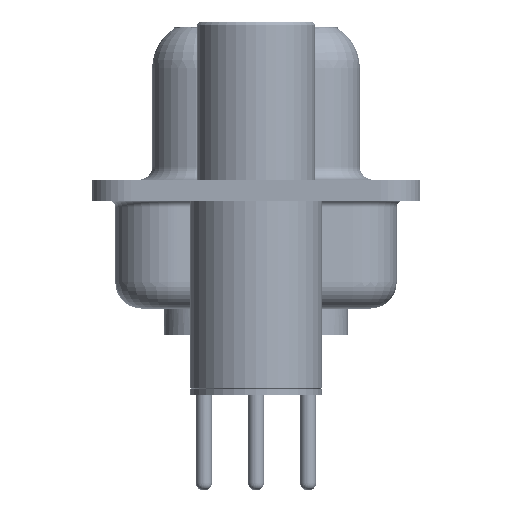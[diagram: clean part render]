
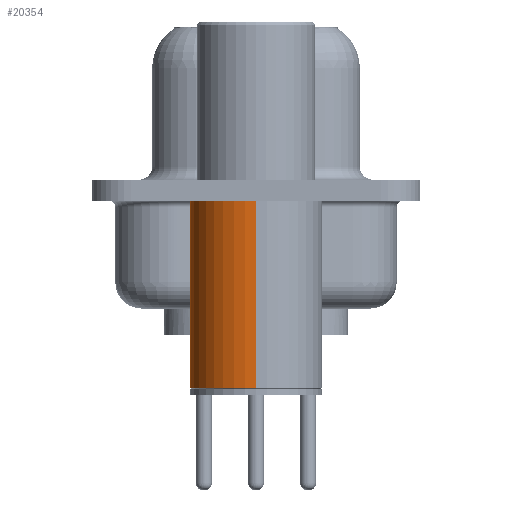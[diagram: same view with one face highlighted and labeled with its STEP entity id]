
A CAD part, left-side view. The second image highlights one B-rep face of the part: STEP entity #20354.
In plain terms, the highlighted cylindrical face has radius 2.5 mm (diameter 5 mm), a partial arc.
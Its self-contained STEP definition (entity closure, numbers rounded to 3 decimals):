
#2364 = ORIENTED_EDGE ( 'NONE', *, *, #29341, .T. ) ;
#3206 = DIRECTION ( 'NONE',  ( 0., 0., 1. ) ) ;
#3695 = EDGE_CURVE ( 'NONE', #34399, #14081, #30120, .T. ) ;
#4918 = CARTESIAN_POINT ( 'NONE',  ( 0., 0., -0.4 ) ) ;
#7027 = CARTESIAN_POINT ( 'NONE',  ( 0., 0., -7.525 ) ) ;
#7965 = ORIENTED_EDGE ( 'NONE', *, *, #10980, .T. ) ;
#7990 = DIRECTION ( 'NONE',  ( 0., 0., 1. ) ) ;
#8004 = DIRECTION ( 'NONE',  ( 0., 0., 1. ) ) ;
#9469 = DIRECTION ( 'NONE',  ( 1., 0., 0. ) ) ;
#10980 = EDGE_CURVE ( 'NONE', #38364, #31230, #26488, .T. ) ;
#11518 = DIRECTION ( 'NONE',  ( 0., 0., 1. ) ) ;
#12091 = CARTESIAN_POINT ( 'NONE',  ( -2.5, 0., -7.525 ) ) ;
#12230 = CARTESIAN_POINT ( 'NONE',  ( 0., 0., 0.581 ) ) ;
#14081 = VERTEX_POINT ( 'NONE', #16760 ) ;
#14703 = CARTESIAN_POINT ( 'NONE',  ( 2.5, 0., -7.525 ) ) ;
#15160 = CARTESIAN_POINT ( 'NONE',  ( 2.5, 0., -0.4 ) ) ;
#16760 = CARTESIAN_POINT ( 'NONE',  ( -2.5, 0., -0.4 ) ) ;
#17499 = ORIENTED_EDGE ( 'NONE', *, *, #38220, .F. ) ;
#17519 = DIRECTION ( 'NONE',  ( 1., 0., 0. ) ) ;
#18242 = ORIENTED_EDGE ( 'NONE', *, *, #3695, .F. ) ;
#18561 = AXIS2_PLACEMENT_3D ( 'NONE', #4918, #11518, #17519 ) ;
#18621 = CYLINDRICAL_SURFACE ( 'NONE', #30318, 2.5 ) ;
#19211 = FACE_OUTER_BOUND ( 'NONE', #22945, .T. ) ;
#20043 = AXIS2_PLACEMENT_3D ( 'NONE', #7027, #28112, #9469 ) ;
#20354 = ADVANCED_FACE ( 'NONE', ( #19211 ), #18621, .T. ) ;
#20602 = LINE ( 'NONE', #23225, #35586 ) ;
#22945 = EDGE_LOOP ( 'NONE', ( #7965, #2364, #18242, #17499 ) ) ;
#23225 = CARTESIAN_POINT ( 'NONE',  ( 2.5, 0., 0.581 ) ) ;
#26488 = CIRCLE ( 'NONE', #20043, 2.5 ) ;
#28112 = DIRECTION ( 'NONE',  ( 0., 0., 1. ) ) ;
#29341 = EDGE_CURVE ( 'NONE', #31230, #14081, #38497, .T. ) ;
#30120 = CIRCLE ( 'NONE', #18561, 2.5 ) ;
#30318 = AXIS2_PLACEMENT_3D ( 'NONE', #12230, #3206, #31279 ) ;
#31230 = VERTEX_POINT ( 'NONE', #12091 ) ;
#31279 = DIRECTION ( 'NONE',  ( 1., 0., 0. ) ) ;
#34399 = VERTEX_POINT ( 'NONE', #15160 ) ;
#35469 = CARTESIAN_POINT ( 'NONE',  ( -2.5, 0., 0.581 ) ) ;
#35586 = VECTOR ( 'NONE', #8004, 1000. ) ;
#36516 = VECTOR ( 'NONE', #7990, 1000. ) ;
#38220 = EDGE_CURVE ( 'NONE', #38364, #34399, #20602, .T. ) ;
#38364 = VERTEX_POINT ( 'NONE', #14703 ) ;
#38497 = LINE ( 'NONE', #35469, #36516 ) ;
